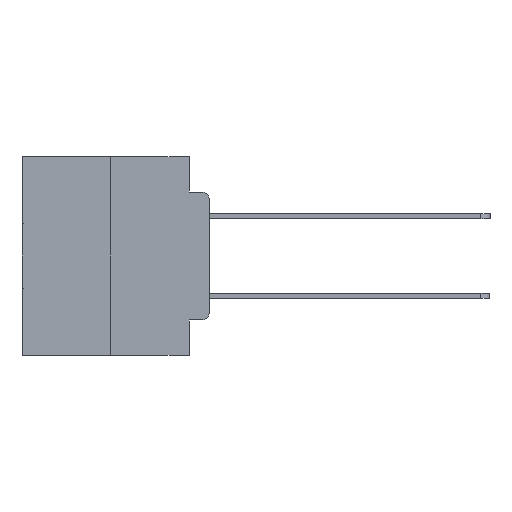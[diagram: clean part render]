
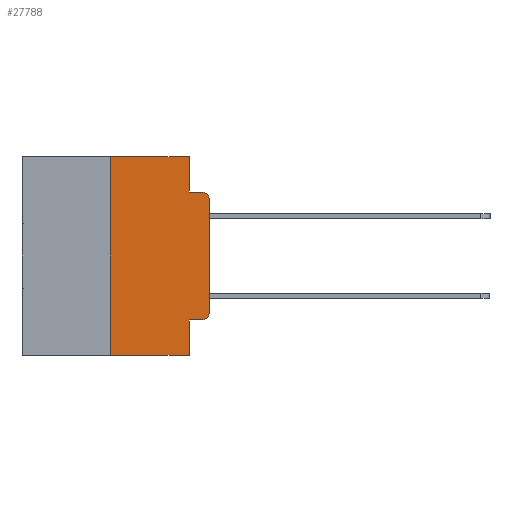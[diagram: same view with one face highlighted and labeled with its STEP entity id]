
A CAD part, left-side view. The second image highlights one B-rep face of the part: STEP entity #27788.
In plain terms, the highlighted planar face has unit normal (-1, 0, 0).
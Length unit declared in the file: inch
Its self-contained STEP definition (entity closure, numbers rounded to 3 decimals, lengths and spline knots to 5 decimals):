
#373 = CARTESIAN_POINT ( 'NONE',  ( 0., 0.051, -0.0885 ) ) ;
#676 = CIRCLE ( 'NONE', #21259, 0.02 ) ;
#1193 = EDGE_CURVE ( 'NONE', #11467, #16784, #10972, .T. ) ;
#2197 = LINE ( 'NONE', #11435, #13653 ) ;
#2366 = ORIENTED_EDGE ( 'NONE', *, *, #1193, .T. ) ;
#2471 = CARTESIAN_POINT ( 'NONE',  ( 0., 0.051, -0.4115 ) ) ;
#3704 = CARTESIAN_POINT ( 'NONE',  ( 0., 0.02, -0.3915 ) ) ;
#4032 = CARTESIAN_POINT ( 'NONE',  ( 0., 0., 0. ) ) ;
#4203 = VECTOR ( 'NONE', #21403, 39.37008 ) ;
#4328 = EDGE_CURVE ( 'NONE', #16784, #19366, #20497, .T. ) ;
#4462 = CARTESIAN_POINT ( 'NONE',  ( 0., 0.051, -0.5 ) ) ;
#4768 = CARTESIAN_POINT ( 'NONE',  ( 0., 0.051, -0.0885 ) ) ;
#4980 = AXIS2_PLACEMENT_3D ( 'NONE', #3704, #19683, #5985 ) ;
#5084 = CARTESIAN_POINT ( 'NONE',  ( 0., 0.25, -0.5 ) ) ;
#5388 = DIRECTION ( 'NONE',  ( 0., 0., 1. ) ) ;
#5640 = VERTEX_POINT ( 'NONE', #29023 ) ;
#5802 = DIRECTION ( 'NONE',  ( 1., 0., 0. ) ) ;
#5985 = DIRECTION ( 'NONE',  ( 0., 0., -1. ) ) ;
#6758 = VERTEX_POINT ( 'NONE', #12840 ) ;
#6957 = CARTESIAN_POINT ( 'NONE',  ( 0., 0.02, -0.4115 ) ) ;
#9352 = VERTEX_POINT ( 'NONE', #4768 ) ;
#9919 = VECTOR ( 'NONE', #5388, 39.37008 ) ;
#10208 = ORIENTED_EDGE ( 'NONE', *, *, #18699, .F. ) ;
#10972 = LINE ( 'NONE', #29302, #4203 ) ;
#11111 = VECTOR ( 'NONE', #24360, 39.37008 ) ;
#11369 = LINE ( 'NONE', #23697, #9919 ) ;
#11435 = CARTESIAN_POINT ( 'NONE',  ( 0., 0.473, -0.5 ) ) ;
#11467 = VERTEX_POINT ( 'NONE', #2471 ) ;
#12108 = VECTOR ( 'NONE', #14160, 39.37008 ) ;
#12545 = EDGE_CURVE ( 'NONE', #19366, #5640, #24077, .T. ) ;
#12584 = PLANE ( 'NONE',  #13391 ) ;
#12840 = CARTESIAN_POINT ( 'NONE',  ( 0., 0.051, 0. ) ) ;
#12958 = CARTESIAN_POINT ( 'NONE',  ( 0., 0.473, 0. ) ) ;
#13101 = ORIENTED_EDGE ( 'NONE', *, *, #27814, .F. ) ;
#13147 = CARTESIAN_POINT ( 'NONE',  ( 0., 0.02, -0.1085 ) ) ;
#13182 = VERTEX_POINT ( 'NONE', #5084 ) ;
#13391 = AXIS2_PLACEMENT_3D ( 'NONE', #23997, #5802, #21808 ) ;
#13653 = VECTOR ( 'NONE', #13827, 39.37008 ) ;
#13827 = DIRECTION ( 'NONE',  ( 0., -1., 0. ) ) ;
#14160 = DIRECTION ( 'NONE',  ( 0., -1., 0. ) ) ;
#14999 = CARTESIAN_POINT ( 'NONE',  ( 0., 0.051, 0. ) ) ;
#15482 = DIRECTION ( 'NONE',  ( 0., 0., -1. ) ) ;
#15630 = ORIENTED_EDGE ( 'NONE', *, *, #12545, .T. ) ;
#15697 = VERTEX_POINT ( 'NONE', #27966 ) ;
#16673 = CARTESIAN_POINT ( 'NONE',  ( 0., 0.25, 0. ) ) ;
#16784 = VERTEX_POINT ( 'NONE', #6957 ) ;
#17071 = ORIENTED_EDGE ( 'NONE', *, *, #21766, .F. ) ;
#17170 = EDGE_CURVE ( 'NONE', #5640, #15697, #676, .T. ) ;
#17295 = VERTEX_POINT ( 'NONE', #4462 ) ;
#17355 = EDGE_CURVE ( 'NONE', #13182, #17295, #2197, .T. ) ;
#17502 = VERTEX_POINT ( 'NONE', #16673 ) ;
#18024 = VECTOR ( 'NONE', #20007, 39.37008 ) ;
#18236 = LINE ( 'NONE', #373, #12108 ) ;
#18496 = ORIENTED_EDGE ( 'NONE', *, *, #24799, .F. ) ;
#18699 = EDGE_CURVE ( 'NONE', #9352, #15697, #18236, .T. ) ;
#19366 = VERTEX_POINT ( 'NONE', #28840 ) ;
#19683 = DIRECTION ( 'NONE',  ( -1., 0., 0. ) ) ;
#20007 = DIRECTION ( 'NONE',  ( 0., 0., 1. ) ) ;
#20157 = LINE ( 'NONE', #23454, #26220 ) ;
#20497 = CIRCLE ( 'NONE', #4980, 0.02 ) ;
#20634 = ORIENTED_EDGE ( 'NONE', *, *, #4328, .T. ) ;
#21259 = AXIS2_PLACEMENT_3D ( 'NONE', #13147, #29066, #15482 ) ;
#21403 = DIRECTION ( 'NONE',  ( 0., -1., 0. ) ) ;
#21513 = EDGE_LOOP ( 'NONE', ( #15630, #27713, #10208, #17071, #29117, #18496, #24548, #13101, #2366, #20634 ) ) ;
#21766 = EDGE_CURVE ( 'NONE', #6758, #9352, #20157, .T. ) ;
#21808 = DIRECTION ( 'NONE',  ( 0., 0., -1. ) ) ;
#21911 = DIRECTION ( 'NONE',  ( 0., 0., -1. ) ) ;
#23043 = VECTOR ( 'NONE', #21911, 39.37008 ) ;
#23239 = EDGE_CURVE ( 'NONE', #17502, #6758, #23304, .T. ) ;
#23304 = LINE ( 'NONE', #12958, #11111 ) ;
#23454 = CARTESIAN_POINT ( 'NONE',  ( 0., 0.051, 0. ) ) ;
#23697 = CARTESIAN_POINT ( 'NONE',  ( 0., 0.25, 0. ) ) ;
#23771 = FACE_OUTER_BOUND ( 'NONE', #21513, .T. ) ;
#23997 = CARTESIAN_POINT ( 'NONE',  ( 0., 0.473, 0. ) ) ;
#24077 = LINE ( 'NONE', #4032, #18024 ) ;
#24360 = DIRECTION ( 'NONE',  ( 0., -1., 0. ) ) ;
#24548 = ORIENTED_EDGE ( 'NONE', *, *, #17355, .T. ) ;
#24799 = EDGE_CURVE ( 'NONE', #13182, #17502, #11369, .T. ) ;
#25732 = DIRECTION ( 'NONE',  ( 0., 0., -1. ) ) ;
#26220 = VECTOR ( 'NONE', #25732, 39.37008 ) ;
#27713 = ORIENTED_EDGE ( 'NONE', *, *, #17170, .T. ) ;
#27788 = ADVANCED_FACE ( 'NONE', ( #23771 ), #12584, .F. ) ;
#27814 = EDGE_CURVE ( 'NONE', #11467, #17295, #29036, .T. ) ;
#27966 = CARTESIAN_POINT ( 'NONE',  ( 0., 0.02, -0.0885 ) ) ;
#28840 = CARTESIAN_POINT ( 'NONE',  ( 0., 0., -0.3915 ) ) ;
#29023 = CARTESIAN_POINT ( 'NONE',  ( 0., 0., -0.1085 ) ) ;
#29036 = LINE ( 'NONE', #14999, #23043 ) ;
#29066 = DIRECTION ( 'NONE',  ( -1., 0., 0. ) ) ;
#29117 = ORIENTED_EDGE ( 'NONE', *, *, #23239, .F. ) ;
#29302 = CARTESIAN_POINT ( 'NONE',  ( 0., 0.051, -0.4115 ) ) ;
